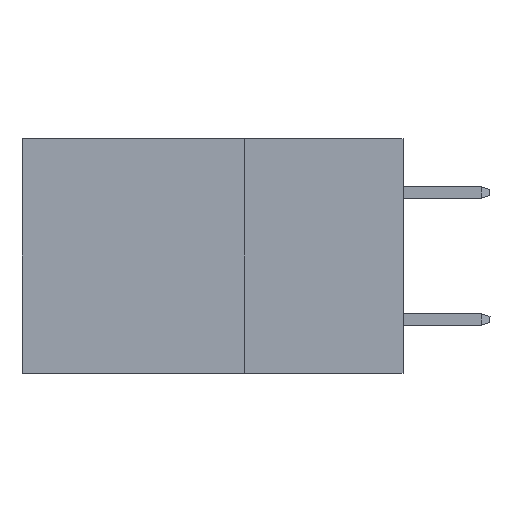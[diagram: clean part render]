
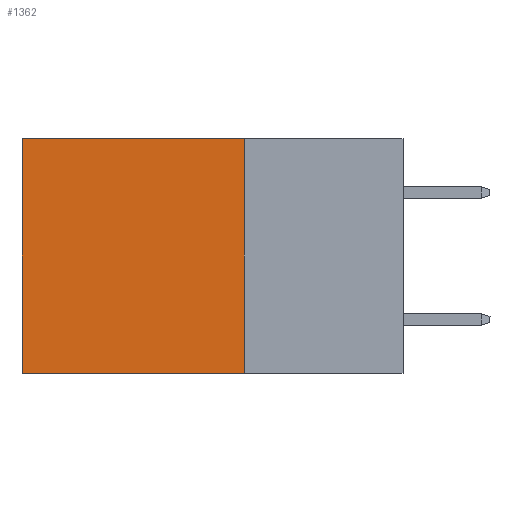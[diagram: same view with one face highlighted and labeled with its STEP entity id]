
A CAD part, left-side view. The second image highlights one B-rep face of the part: STEP entity #1362.
In plain terms, the highlighted planar face has unit normal (-1, 0, 0).
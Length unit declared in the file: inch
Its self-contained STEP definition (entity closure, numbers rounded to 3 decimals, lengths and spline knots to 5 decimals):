
#384 = CARTESIAN_POINT ( 'NONE',  ( 0.2875, 0.25, 0. ) ) ;
#562 = VERTEX_POINT ( 'NONE', #3034 ) ;
#604 = ORIENTED_EDGE ( 'NONE', *, *, #2879, .T. ) ;
#672 = CARTESIAN_POINT ( 'NONE',  ( 0.2875, 0.6, 0. ) ) ;
#895 = VECTOR ( 'NONE', #5120, 39.37008 ) ;
#925 = DIRECTION ( 'NONE',  ( 0., 1., 0. ) ) ;
#1362 = ADVANCED_FACE ( 'NONE', ( #10098 ), #9315, .F. ) ;
#2296 = CARTESIAN_POINT ( 'NONE',  ( 0.2875, 0.6, -0.37 ) ) ;
#2376 = AXIS2_PLACEMENT_3D ( 'NONE', #8539, #10156, #3108 ) ;
#2501 = EDGE_CURVE ( 'NONE', #8896, #562, #2626, .T. ) ;
#2626 = LINE ( 'NONE', #384, #895 ) ;
#2879 = EDGE_CURVE ( 'NONE', #8896, #10017, #7165, .T. ) ;
#3034 = CARTESIAN_POINT ( 'NONE',  ( 0.2875, 0.25, -0.37 ) ) ;
#3108 = DIRECTION ( 'NONE',  ( 0., 0., -1. ) ) ;
#3178 = EDGE_CURVE ( 'NONE', #562, #4383, #7202, .T. ) ;
#3686 = VECTOR ( 'NONE', #9488, 39.37008 ) ;
#4383 = VERTEX_POINT ( 'NONE', #2296 ) ;
#4431 = EDGE_CURVE ( 'NONE', #10017, #4383, #6239, .T. ) ;
#5120 = DIRECTION ( 'NONE',  ( 0., 0., -1. ) ) ;
#5622 = CARTESIAN_POINT ( 'NONE',  ( 0.2875, 0.25, 0. ) ) ;
#6139 = DIRECTION ( 'NONE',  ( 0., 0., -1. ) ) ;
#6239 = LINE ( 'NONE', #8617, #7431 ) ;
#7165 = LINE ( 'NONE', #5622, #3686 ) ;
#7202 = LINE ( 'NONE', #8424, #7236 ) ;
#7236 = VECTOR ( 'NONE', #925, 39.37008 ) ;
#7431 = VECTOR ( 'NONE', #6139, 39.37008 ) ;
#7483 = CARTESIAN_POINT ( 'NONE',  ( 0.2875, 0.25, 0. ) ) ;
#7589 = ORIENTED_EDGE ( 'NONE', *, *, #4431, .T. ) ;
#8424 = CARTESIAN_POINT ( 'NONE',  ( 0.2875, 0.25, -0.37 ) ) ;
#8539 = CARTESIAN_POINT ( 'NONE',  ( 0.2875, 0.25, 0. ) ) ;
#8617 = CARTESIAN_POINT ( 'NONE',  ( 0.2875, 0.6, 0. ) ) ;
#8795 = ORIENTED_EDGE ( 'NONE', *, *, #2501, .F. ) ;
#8896 = VERTEX_POINT ( 'NONE', #7483 ) ;
#9234 = ORIENTED_EDGE ( 'NONE', *, *, #3178, .F. ) ;
#9315 = PLANE ( 'NONE',  #2376 ) ;
#9488 = DIRECTION ( 'NONE',  ( 0., 1., 0. ) ) ;
#9524 = EDGE_LOOP ( 'NONE', ( #7589, #9234, #8795, #604 ) ) ;
#10017 = VERTEX_POINT ( 'NONE', #672 ) ;
#10098 = FACE_OUTER_BOUND ( 'NONE', #9524, .T. ) ;
#10156 = DIRECTION ( 'NONE',  ( 1., 0., 0. ) ) ;
